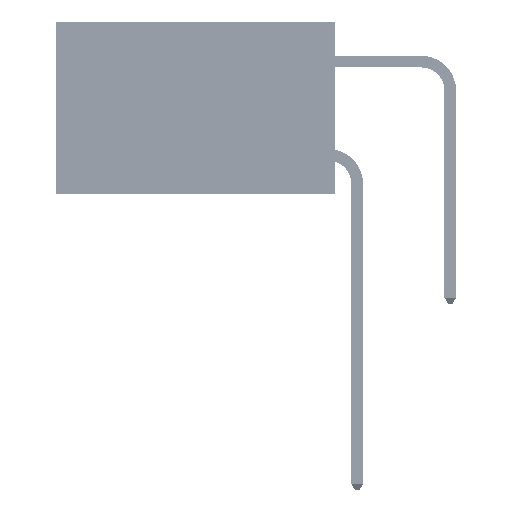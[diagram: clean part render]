
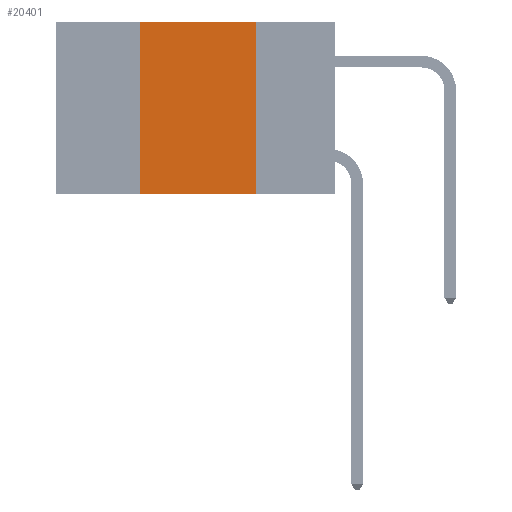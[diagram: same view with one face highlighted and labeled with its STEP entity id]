
A CAD part, left-side view. The second image highlights one B-rep face of the part: STEP entity #20401.
In plain terms, the highlighted planar face has unit normal (-1, 0, 0).
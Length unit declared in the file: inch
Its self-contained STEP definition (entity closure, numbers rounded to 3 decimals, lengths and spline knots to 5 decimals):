
#681 = DIRECTION ( 'NONE',  ( 0., 0., 1. ) ) ;
#2456 = ORIENTED_EDGE ( 'NONE', *, *, #41527, .F. ) ;
#3987 = DIRECTION ( 'NONE',  ( 0., 0., -1. ) ) ;
#4314 = DIRECTION ( 'NONE',  ( 0., 0., -1. ) ) ;
#5071 = LINE ( 'NONE', #45142, #34452 ) ;
#7326 = VERTEX_POINT ( 'NONE', #37299 ) ;
#8000 = DIRECTION ( 'NONE',  ( 1., 0., 0. ) ) ;
#8839 = VERTEX_POINT ( 'NONE', #11868 ) ;
#8877 = VECTOR ( 'NONE', #3987, 39.37008 ) ;
#9481 = LINE ( 'NONE', #15221, #8877 ) ;
#9484 = ORIENTED_EDGE ( 'NONE', *, *, #16629, .F. ) ;
#10490 = ORIENTED_EDGE ( 'NONE', *, *, #32975, .T. ) ;
#11868 = CARTESIAN_POINT ( 'NONE',  ( 0., 0.17, -0.37 ) ) ;
#11913 = CARTESIAN_POINT ( 'NONE',  ( 0., 0.42, 0. ) ) ;
#15221 = CARTESIAN_POINT ( 'NONE',  ( 0., 0.17, 0. ) ) ;
#16629 = EDGE_CURVE ( 'NONE', #38544, #33517, #5071, .T. ) ;
#17892 = VECTOR ( 'NONE', #42302, 39.37008 ) ;
#20401 = ADVANCED_FACE ( 'NONE', ( #46452 ), #22976, .F. ) ;
#22976 = PLANE ( 'NONE',  #44130 ) ;
#26839 = CARTESIAN_POINT ( 'NONE',  ( 0., 0.6, 0. ) ) ;
#27234 = LINE ( 'NONE', #11913, #27804 ) ;
#27804 = VECTOR ( 'NONE', #681, 39.37008 ) ;
#28787 = EDGE_CURVE ( 'NONE', #7326, #38544, #27234, .T. ) ;
#31142 = CARTESIAN_POINT ( 'NONE',  ( 0., 0.42, 0. ) ) ;
#31163 = LINE ( 'NONE', #45683, #17892 ) ;
#32975 = EDGE_CURVE ( 'NONE', #7326, #8839, #31163, .T. ) ;
#33441 = DIRECTION ( 'NONE',  ( 0., -1., 0. ) ) ;
#33517 = VERTEX_POINT ( 'NONE', #38231 ) ;
#34452 = VECTOR ( 'NONE', #33441, 39.37008 ) ;
#37299 = CARTESIAN_POINT ( 'NONE',  ( 0., 0.42, -0.37 ) ) ;
#38231 = CARTESIAN_POINT ( 'NONE',  ( 0., 0.17, 0. ) ) ;
#38544 = VERTEX_POINT ( 'NONE', #31142 ) ;
#41527 = EDGE_CURVE ( 'NONE', #33517, #8839, #9481, .T. ) ;
#42302 = DIRECTION ( 'NONE',  ( 0., -1., 0. ) ) ;
#44130 = AXIS2_PLACEMENT_3D ( 'NONE', #26839, #8000, #4314 ) ;
#44796 = EDGE_LOOP ( 'NONE', ( #2456, #9484, #46390, #10490 ) ) ;
#45142 = CARTESIAN_POINT ( 'NONE',  ( 0., 0.6, 0. ) ) ;
#45683 = CARTESIAN_POINT ( 'NONE',  ( 0., 0.6, -0.37 ) ) ;
#46390 = ORIENTED_EDGE ( 'NONE', *, *, #28787, .F. ) ;
#46452 = FACE_OUTER_BOUND ( 'NONE', #44796, .T. ) ;
